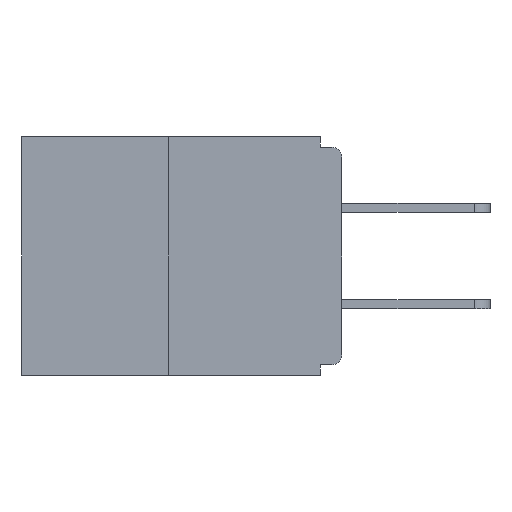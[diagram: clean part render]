
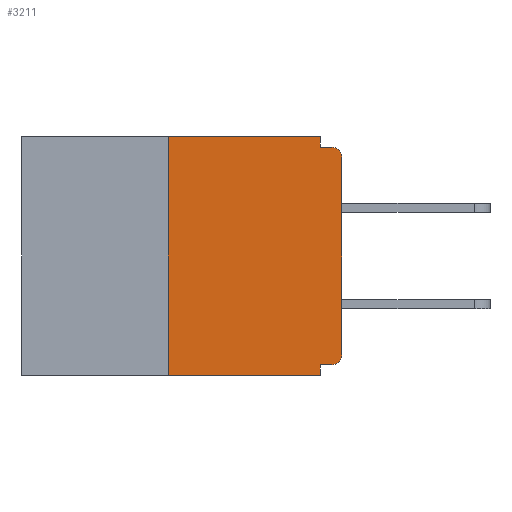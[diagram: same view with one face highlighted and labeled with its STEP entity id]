
A CAD part, left-side view. The second image highlights one B-rep face of the part: STEP entity #3211.
In plain terms, the highlighted planar face has unit normal (-1, 0, 0).
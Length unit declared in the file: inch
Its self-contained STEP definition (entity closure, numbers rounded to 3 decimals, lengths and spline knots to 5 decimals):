
#422 = AXIS2_PLACEMENT_3D ( 'NONE', #24673, #27576, #18157 ) ;
#532 = CARTESIAN_POINT ( 'NONE',  ( 0., 0.25, 0. ) ) ;
#1831 = DIRECTION ( 'NONE',  ( 0., 1., 0. ) ) ;
#1986 = ORIENTED_EDGE ( 'NONE', *, *, #2496, .F. ) ;
#2310 = LINE ( 'NONE', #30083, #21811 ) ;
#2496 = EDGE_CURVE ( 'NONE', #8582, #22263, #15994, .T. ) ;
#2823 = CARTESIAN_POINT ( 'NONE',  ( 0., 0.46, 0. ) ) ;
#3211 = ADVANCED_FACE ( 'NONE', ( #12131 ), #19340, .F. ) ;
#3866 = EDGE_CURVE ( 'NONE', #20112, #20698, #21945, .T. ) ;
#3877 = ORIENTED_EDGE ( 'NONE', *, *, #6466, .T. ) ;
#4739 = CARTESIAN_POINT ( 'NONE',  ( 0., 0.031, 0. ) ) ;
#5031 = CARTESIAN_POINT ( 'NONE',  ( 0., 0.031, -0.015 ) ) ;
#5042 = ORIENTED_EDGE ( 'NONE', *, *, #3866, .F. ) ;
#5266 = AXIS2_PLACEMENT_3D ( 'NONE', #10532, #17904, #6046 ) ;
#5932 = ORIENTED_EDGE ( 'NONE', *, *, #10787, .T. ) ;
#6046 = DIRECTION ( 'NONE',  ( 0., 0., -1. ) ) ;
#6220 = VECTOR ( 'NONE', #30851, 39.37008 ) ;
#6466 = EDGE_CURVE ( 'NONE', #7773, #22263, #17253, .T. ) ;
#6508 = CIRCLE ( 'NONE', #5266, 0.015 ) ;
#7056 = VERTEX_POINT ( 'NONE', #11299 ) ;
#7150 = CARTESIAN_POINT ( 'NONE',  ( 0., 0.25, 0. ) ) ;
#7569 = DIRECTION ( 'NONE',  ( 0., 0., 1. ) ) ;
#7697 = DIRECTION ( 'NONE',  ( 0., -1., 0. ) ) ;
#7740 = EDGE_LOOP ( 'NONE', ( #17889, #28553, #3877, #1986, #21795, #24413, #5932, #24764, #5042, #17271 ) ) ;
#7773 = VERTEX_POINT ( 'NONE', #11248 ) ;
#8582 = VERTEX_POINT ( 'NONE', #16970 ) ;
#10532 = CARTESIAN_POINT ( 'NONE',  ( 0., 0.015, -0.313 ) ) ;
#10787 = EDGE_CURVE ( 'NONE', #30218, #7056, #27510, .T. ) ;
#11248 = CARTESIAN_POINT ( 'NONE',  ( 0., 0.25, -0.343 ) ) ;
#11299 = CARTESIAN_POINT ( 'NONE',  ( 0., 0., -0.03 ) ) ;
#11380 = DIRECTION ( 'NONE',  ( -1., 0., 0. ) ) ;
#11457 = AXIS2_PLACEMENT_3D ( 'NONE', #25770, #11380, #30541 ) ;
#11597 = CARTESIAN_POINT ( 'NONE',  ( 0., 0., 0. ) ) ;
#12131 = FACE_OUTER_BOUND ( 'NONE', #7740, .T. ) ;
#12148 = EDGE_CURVE ( 'NONE', #22994, #30218, #6508, .T. ) ;
#14023 = VECTOR ( 'NONE', #16965, 39.37008 ) ;
#14351 = EDGE_CURVE ( 'NONE', #7773, #15276, #16197, .T. ) ;
#14658 = VECTOR ( 'NONE', #7569, 39.37008 ) ;
#15276 = VERTEX_POINT ( 'NONE', #7150 ) ;
#15773 = CARTESIAN_POINT ( 'NONE',  ( 0., 0.031, -0.343 ) ) ;
#15842 = CARTESIAN_POINT ( 'NONE',  ( 0., 0., -0.015 ) ) ;
#15994 = LINE ( 'NONE', #16657, #6220 ) ;
#16197 = LINE ( 'NONE', #532, #14658 ) ;
#16476 = DIRECTION ( 'NONE',  ( 0., 0., 1. ) ) ;
#16653 = VECTOR ( 'NONE', #16476, 39.37008 ) ;
#16657 = CARTESIAN_POINT ( 'NONE',  ( 0., 0.031, -0.343 ) ) ;
#16929 = CARTESIAN_POINT ( 'NONE',  ( 0., 0.015, -0.328 ) ) ;
#16965 = DIRECTION ( 'NONE',  ( 0., -1., 0. ) ) ;
#16970 = CARTESIAN_POINT ( 'NONE',  ( 0., 0.031, -0.328 ) ) ;
#17182 = CARTESIAN_POINT ( 'NONE',  ( 0., 0.46, -0.343 ) ) ;
#17253 = LINE ( 'NONE', #17182, #19172 ) ;
#17271 = ORIENTED_EDGE ( 'NONE', *, *, #25477, .F. ) ;
#17323 = CARTESIAN_POINT ( 'NONE',  ( 0., 0., -0.313 ) ) ;
#17889 = ORIENTED_EDGE ( 'NONE', *, *, #29619, .F. ) ;
#17904 = DIRECTION ( 'NONE',  ( -1., 0., 0. ) ) ;
#18157 = DIRECTION ( 'NONE',  ( 0., 0., -1. ) ) ;
#18282 = DIRECTION ( 'NONE',  ( 0., 0., -1. ) ) ;
#19172 = VECTOR ( 'NONE', #7697, 39.37008 ) ;
#19340 = PLANE ( 'NONE',  #422 ) ;
#20112 = VERTEX_POINT ( 'NONE', #5031 ) ;
#20261 = CARTESIAN_POINT ( 'NONE',  ( 0., 0.015, -0.015 ) ) ;
#20426 = VECTOR ( 'NONE', #1831, 39.37008 ) ;
#20698 = VERTEX_POINT ( 'NONE', #20261 ) ;
#21017 = EDGE_CURVE ( 'NONE', #22994, #8582, #24494, .T. ) ;
#21078 = EDGE_CURVE ( 'NONE', #7056, #20698, #25243, .T. ) ;
#21554 = LINE ( 'NONE', #2823, #14023 ) ;
#21795 = ORIENTED_EDGE ( 'NONE', *, *, #21017, .F. ) ;
#21811 = VECTOR ( 'NONE', #18282, 39.37008 ) ;
#21945 = LINE ( 'NONE', #15842, #26058 ) ;
#22263 = VERTEX_POINT ( 'NONE', #15773 ) ;
#22994 = VERTEX_POINT ( 'NONE', #16929 ) ;
#24413 = ORIENTED_EDGE ( 'NONE', *, *, #12148, .T. ) ;
#24494 = LINE ( 'NONE', #28066, #20426 ) ;
#24673 = CARTESIAN_POINT ( 'NONE',  ( 0., 0.46, 0. ) ) ;
#24764 = ORIENTED_EDGE ( 'NONE', *, *, #21078, .T. ) ;
#25243 = CIRCLE ( 'NONE', #11457, 0.015 ) ;
#25477 = EDGE_CURVE ( 'NONE', #26906, #20112, #2310, .T. ) ;
#25770 = CARTESIAN_POINT ( 'NONE',  ( 0., 0.015, -0.03 ) ) ;
#26058 = VECTOR ( 'NONE', #30336, 39.37008 ) ;
#26906 = VERTEX_POINT ( 'NONE', #4739 ) ;
#27510 = LINE ( 'NONE', #11597, #16653 ) ;
#27576 = DIRECTION ( 'NONE',  ( 1., 0., 0. ) ) ;
#28066 = CARTESIAN_POINT ( 'NONE',  ( 0., 0., -0.328 ) ) ;
#28553 = ORIENTED_EDGE ( 'NONE', *, *, #14351, .F. ) ;
#29619 = EDGE_CURVE ( 'NONE', #15276, #26906, #21554, .T. ) ;
#30083 = CARTESIAN_POINT ( 'NONE',  ( 0., 0.031, 0. ) ) ;
#30218 = VERTEX_POINT ( 'NONE', #17323 ) ;
#30336 = DIRECTION ( 'NONE',  ( 0., -1., 0. ) ) ;
#30541 = DIRECTION ( 'NONE',  ( 0., 0., -1. ) ) ;
#30851 = DIRECTION ( 'NONE',  ( 0., 0., -1. ) ) ;
